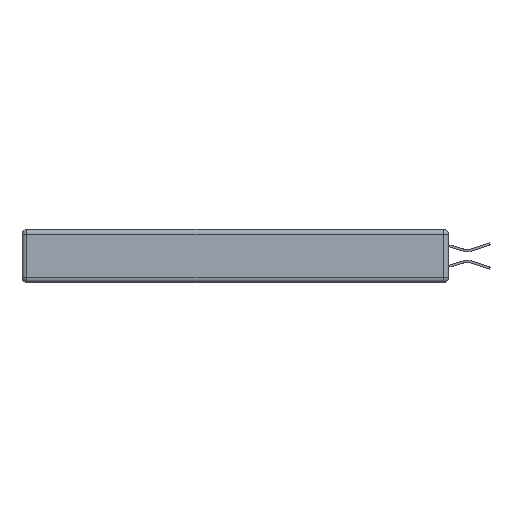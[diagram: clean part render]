
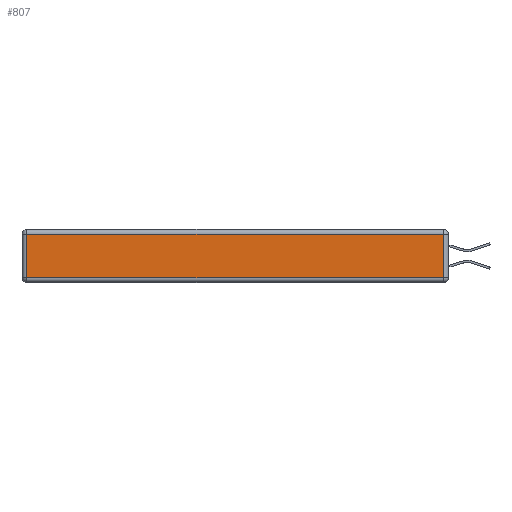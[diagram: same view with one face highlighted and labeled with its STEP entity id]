
A CAD part, left-side view. The second image highlights one B-rep face of the part: STEP entity #807.
In plain terms, the highlighted planar face has unit normal (-1, 0, 0).
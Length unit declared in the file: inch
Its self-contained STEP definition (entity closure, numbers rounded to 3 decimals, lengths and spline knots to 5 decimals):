
#587 = DIRECTION ( 'NONE',  ( 0., 1., 0. ) ) ;
#618 = AXIS2_PLACEMENT_3D ( 'NONE', #16145, #9705, #14866 ) ;
#807 = ADVANCED_FACE ( 'NONE', ( #5114 ), #13595, .T. ) ;
#1122 = DIRECTION ( 'NONE',  ( 0., 0., 1. ) ) ;
#1211 = DIRECTION ( 'NONE',  ( 0., 0., -1. ) ) ;
#1407 = CARTESIAN_POINT ( 'NONE',  ( 0., 2.72, -0.343 ) ) ;
#1738 = LINE ( 'NONE', #13846, #15245 ) ;
#2565 = VERTEX_POINT ( 'NONE', #13261 ) ;
#4655 = DIRECTION ( 'NONE',  ( 0., -1., 0. ) ) ;
#5114 = FACE_OUTER_BOUND ( 'NONE', #8092, .T. ) ;
#5321 = CARTESIAN_POINT ( 'NONE',  ( 0., 2.72, -0.03 ) ) ;
#6394 = LINE ( 'NONE', #9878, #11200 ) ;
#6547 = VERTEX_POINT ( 'NONE', #5321 ) ;
#7955 = ORIENTED_EDGE ( 'NONE', *, *, #14961, .T. ) ;
#8008 = LINE ( 'NONE', #1407, #12984 ) ;
#8053 = VERTEX_POINT ( 'NONE', #14955 ) ;
#8092 = EDGE_LOOP ( 'NONE', ( #16282, #7955, #16841, #13721 ) ) ;
#8252 = EDGE_CURVE ( 'NONE', #16686, #6547, #6394, .T. ) ;
#9247 = LINE ( 'NONE', #16840, #16521 ) ;
#9705 = DIRECTION ( 'NONE',  ( -1., 0., 0. ) ) ;
#9878 = CARTESIAN_POINT ( 'NONE',  ( 0., 2.75, -0.03 ) ) ;
#11200 = VECTOR ( 'NONE', #587, 39.37008 ) ;
#12984 = VECTOR ( 'NONE', #1211, 39.37008 ) ;
#13261 = CARTESIAN_POINT ( 'NONE',  ( 0., 0.03, -0.313 ) ) ;
#13595 = PLANE ( 'NONE',  #618 ) ;
#13721 = ORIENTED_EDGE ( 'NONE', *, *, #14863, .T. ) ;
#13846 = CARTESIAN_POINT ( 'NONE',  ( 0., 0., -0.313 ) ) ;
#13937 = CARTESIAN_POINT ( 'NONE',  ( 0., 0.03, -0.03 ) ) ;
#14863 = EDGE_CURVE ( 'NONE', #6547, #8053, #8008, .T. ) ;
#14866 = DIRECTION ( 'NONE',  ( 0., 0., 1. ) ) ;
#14955 = CARTESIAN_POINT ( 'NONE',  ( 0., 2.72, -0.313 ) ) ;
#14961 = EDGE_CURVE ( 'NONE', #2565, #16686, #9247, .T. ) ;
#15245 = VECTOR ( 'NONE', #4655, 39.37008 ) ;
#15322 = EDGE_CURVE ( 'NONE', #8053, #2565, #1738, .T. ) ;
#16145 = CARTESIAN_POINT ( 'NONE',  ( 0., 0., -0.343 ) ) ;
#16282 = ORIENTED_EDGE ( 'NONE', *, *, #15322, .T. ) ;
#16521 = VECTOR ( 'NONE', #1122, 39.37008 ) ;
#16686 = VERTEX_POINT ( 'NONE', #13937 ) ;
#16840 = CARTESIAN_POINT ( 'NONE',  ( 0., 0.03, -0.343 ) ) ;
#16841 = ORIENTED_EDGE ( 'NONE', *, *, #8252, .T. ) ;
